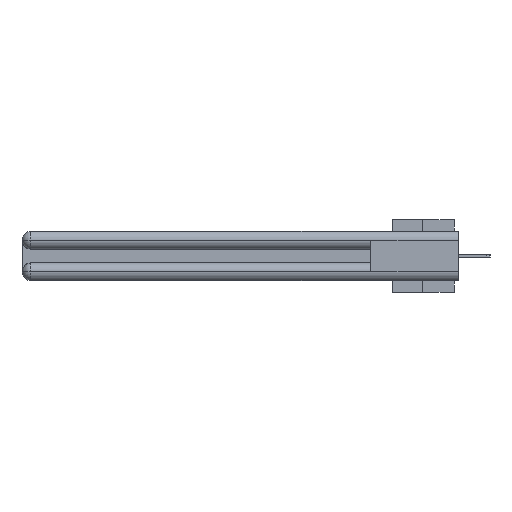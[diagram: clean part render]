
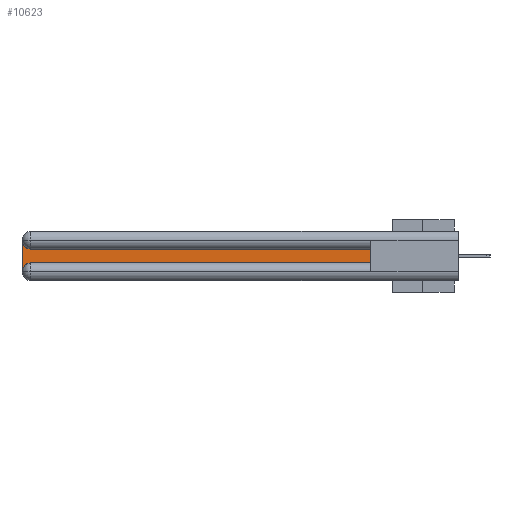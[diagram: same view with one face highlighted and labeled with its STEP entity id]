
A CAD part, left-side view. The second image highlights one B-rep face of the part: STEP entity #10623.
In plain terms, the highlighted planar face has unit normal (-1, 0, 0).
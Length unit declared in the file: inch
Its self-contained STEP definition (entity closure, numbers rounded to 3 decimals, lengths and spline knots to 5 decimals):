
#142 = CARTESIAN_POINT ( 'NONE',  ( 0.075, 3., -0.2775 ) ) ;
#895 = FACE_OUTER_BOUND ( 'NONE', #15468, .T. ) ;
#1143 = AXIS2_PLACEMENT_3D ( 'NONE', #35976, #6494, #39421 ) ;
#1273 = CARTESIAN_POINT ( 'NONE',  ( 0.075, 0.6, -0.2175 ) ) ;
#2106 = CARTESIAN_POINT ( 'NONE',  ( 0.075, 0.6, -0.1225 ) ) ;
#2173 = VERTEX_POINT ( 'NONE', #30882 ) ;
#3642 = CARTESIAN_POINT ( 'NONE',  ( 0.075, 0.6, -0.2175 ) ) ;
#4138 = CARTESIAN_POINT ( 'NONE',  ( 0.075, 2.94, -0.1225 ) ) ;
#5671 = VECTOR ( 'NONE', #14360, 39.37008 ) ;
#5707 = ORIENTED_EDGE ( 'NONE', *, *, #22159, .T. ) ;
#6209 = CARTESIAN_POINT ( 'NONE',  ( 0.075, 2.94, -0.0625 ) ) ;
#6494 = DIRECTION ( 'NONE',  ( 1., 0., 0. ) ) ;
#6870 = EDGE_CURVE ( 'NONE', #21184, #36200, #31146, .T. ) ;
#8271 = DIRECTION ( 'NONE',  ( 0., 0., -1. ) ) ;
#10168 = DIRECTION ( 'NONE',  ( 0., -1., 0. ) ) ;
#10623 = ADVANCED_FACE ( 'NONE', ( #895 ), #26724, .F. ) ;
#11518 = ORIENTED_EDGE ( 'NONE', *, *, #6870, .T. ) ;
#14360 = DIRECTION ( 'NONE',  ( 0., 0., 1. ) ) ;
#15468 = EDGE_LOOP ( 'NONE', ( #5707, #21543, #30077, #16736, #27838, #11518 ) ) ;
#15751 = VERTEX_POINT ( 'NONE', #4138 ) ;
#16392 = DIRECTION ( 'NONE',  ( 0., 0., -1. ) ) ;
#16736 = ORIENTED_EDGE ( 'NONE', *, *, #18644, .T. ) ;
#18156 = VECTOR ( 'NONE', #41356, 39.37008 ) ;
#18644 = EDGE_CURVE ( 'NONE', #36527, #40301, #37585, .T. ) ;
#21147 = CARTESIAN_POINT ( 'NONE',  ( 0.075, 0.6, -0.1225 ) ) ;
#21184 = VERTEX_POINT ( 'NONE', #3642 ) ;
#21543 = ORIENTED_EDGE ( 'NONE', *, *, #22721, .T. ) ;
#22159 = EDGE_CURVE ( 'NONE', #36200, #15751, #40533, .T. ) ;
#22721 = EDGE_CURVE ( 'NONE', #15751, #2173, #24370, .T. ) ;
#22831 = DIRECTION ( 'NONE',  ( 1., 0., 0. ) ) ;
#23698 = CARTESIAN_POINT ( 'NONE',  ( 0.075, 3., -0.1225 ) ) ;
#24370 = CIRCLE ( 'NONE', #28489, 0.06 ) ;
#26013 = DIRECTION ( 'NONE',  ( 1., 0., 0. ) ) ;
#26465 = EDGE_CURVE ( 'NONE', #2173, #36527, #37775, .T. ) ;
#26724 = PLANE ( 'NONE',  #39599 ) ;
#27638 = CARTESIAN_POINT ( 'NONE',  ( 0.075, 2.94, -0.2175 ) ) ;
#27838 = ORIENTED_EDGE ( 'NONE', *, *, #28465, .T. ) ;
#27884 = VECTOR ( 'NONE', #10168, 39.37008 ) ;
#27975 = VECTOR ( 'NONE', #8271, 39.37008 ) ;
#28465 = EDGE_CURVE ( 'NONE', #40301, #21184, #39053, .T. ) ;
#28489 = AXIS2_PLACEMENT_3D ( 'NONE', #6209, #26013, #41946 ) ;
#29324 = CARTESIAN_POINT ( 'NONE',  ( 0.075, 0.6, -0.2175 ) ) ;
#30077 = ORIENTED_EDGE ( 'NONE', *, *, #26465, .T. ) ;
#30882 = CARTESIAN_POINT ( 'NONE',  ( 0.075, 3., -0.0625 ) ) ;
#31146 = LINE ( 'NONE', #1273, #5671 ) ;
#35976 = CARTESIAN_POINT ( 'NONE',  ( 0.075, 2.94, -0.2775 ) ) ;
#36200 = VERTEX_POINT ( 'NONE', #2106 ) ;
#36527 = VERTEX_POINT ( 'NONE', #142 ) ;
#37585 = CIRCLE ( 'NONE', #1143, 0.06 ) ;
#37775 = LINE ( 'NONE', #41204, #27975 ) ;
#39053 = LINE ( 'NONE', #29324, #27884 ) ;
#39421 = DIRECTION ( 'NONE',  ( 0., 0., -1. ) ) ;
#39599 = AXIS2_PLACEMENT_3D ( 'NONE', #23698, #22831, #16392 ) ;
#40301 = VERTEX_POINT ( 'NONE', #27638 ) ;
#40533 = LINE ( 'NONE', #21147, #18156 ) ;
#41204 = CARTESIAN_POINT ( 'NONE',  ( 0.075, 3., -0.2175 ) ) ;
#41356 = DIRECTION ( 'NONE',  ( 0., 1., 0. ) ) ;
#41946 = DIRECTION ( 'NONE',  ( 0., 0., -1. ) ) ;
